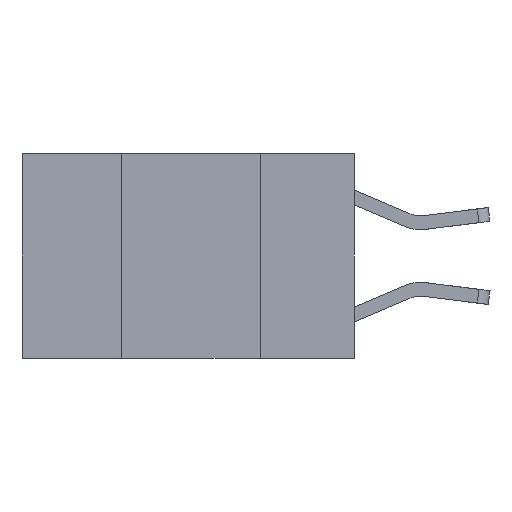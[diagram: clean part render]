
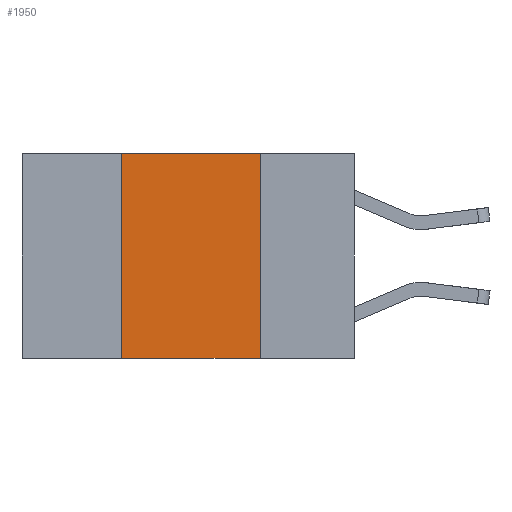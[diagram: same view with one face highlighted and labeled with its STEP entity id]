
A CAD part, left-side view. The second image highlights one B-rep face of the part: STEP entity #1950.
In plain terms, the highlighted planar face has unit normal (-1, 0, 0).
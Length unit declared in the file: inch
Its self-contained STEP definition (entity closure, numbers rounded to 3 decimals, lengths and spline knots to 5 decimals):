
#111 = ORIENTED_EDGE ( 'NONE', *, *, #6556, .F. ) ;
#194 = CARTESIAN_POINT ( 'NONE',  ( 0., 0.17, -0.37 ) ) ;
#410 = CARTESIAN_POINT ( 'NONE',  ( 0., 0.42, -0.37 ) ) ;
#663 = EDGE_CURVE ( 'NONE', #4963, #5161, #5367, .T. ) ;
#695 = CARTESIAN_POINT ( 'NONE',  ( 0., 0.17, 0. ) ) ;
#944 = ORIENTED_EDGE ( 'NONE', *, *, #663, .T. ) ;
#1128 = VECTOR ( 'NONE', #2997, 39.37008 ) ;
#1232 = ORIENTED_EDGE ( 'NONE', *, *, #3580, .F. ) ;
#1645 = EDGE_LOOP ( 'NONE', ( #111, #3923, #1232, #944 ) ) ;
#1771 = CARTESIAN_POINT ( 'NONE',  ( 0., 0.6, -0.37 ) ) ;
#1950 = ADVANCED_FACE ( 'NONE', ( #1954 ), #9024, .F. ) ;
#1954 = FACE_OUTER_BOUND ( 'NONE', #1645, .T. ) ;
#2282 = VERTEX_POINT ( 'NONE', #2746 ) ;
#2746 = CARTESIAN_POINT ( 'NONE',  ( 0., 0.42, 0. ) ) ;
#2997 = DIRECTION ( 'NONE',  ( 0., -1., 0. ) ) ;
#3008 = CARTESIAN_POINT ( 'NONE',  ( 0., 0.6, 0. ) ) ;
#3580 = EDGE_CURVE ( 'NONE', #4963, #2282, #6316, .T. ) ;
#3923 = ORIENTED_EDGE ( 'NONE', *, *, #4369, .F. ) ;
#4315 = AXIS2_PLACEMENT_3D ( 'NONE', #8982, #4730, #8191 ) ;
#4369 = EDGE_CURVE ( 'NONE', #2282, #5592, #7035, .T. ) ;
#4527 = VECTOR ( 'NONE', #6246, 39.37008 ) ;
#4537 = CARTESIAN_POINT ( 'NONE',  ( 0., 0.17, 0. ) ) ;
#4730 = DIRECTION ( 'NONE',  ( 1., 0., 0. ) ) ;
#4963 = VERTEX_POINT ( 'NONE', #410 ) ;
#5161 = VERTEX_POINT ( 'NONE', #194 ) ;
#5367 = LINE ( 'NONE', #1771, #8701 ) ;
#5592 = VERTEX_POINT ( 'NONE', #4537 ) ;
#5767 = DIRECTION ( 'NONE',  ( 0., 0., -1. ) ) ;
#6246 = DIRECTION ( 'NONE',  ( 0., 0., 1. ) ) ;
#6294 = CARTESIAN_POINT ( 'NONE',  ( 0., 0.42, 0. ) ) ;
#6316 = LINE ( 'NONE', #6294, #4527 ) ;
#6556 = EDGE_CURVE ( 'NONE', #5592, #5161, #7320, .T. ) ;
#7035 = LINE ( 'NONE', #3008, #1128 ) ;
#7116 = VECTOR ( 'NONE', #5767, 39.37008 ) ;
#7320 = LINE ( 'NONE', #695, #7116 ) ;
#8191 = DIRECTION ( 'NONE',  ( 0., 0., -1. ) ) ;
#8701 = VECTOR ( 'NONE', #8835, 39.37008 ) ;
#8835 = DIRECTION ( 'NONE',  ( 0., -1., 0. ) ) ;
#8982 = CARTESIAN_POINT ( 'NONE',  ( 0., 0.6, 0. ) ) ;
#9024 = PLANE ( 'NONE',  #4315 ) ;
